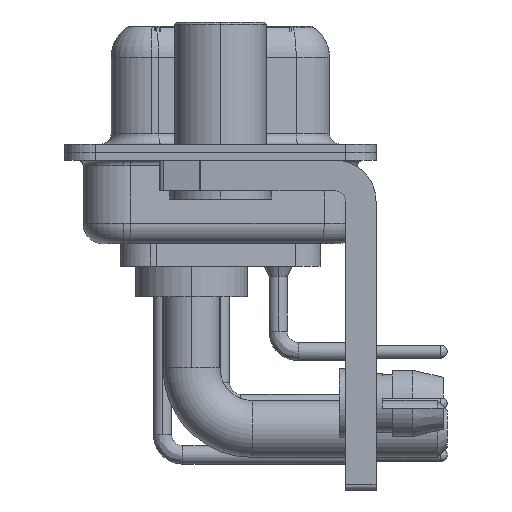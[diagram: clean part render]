
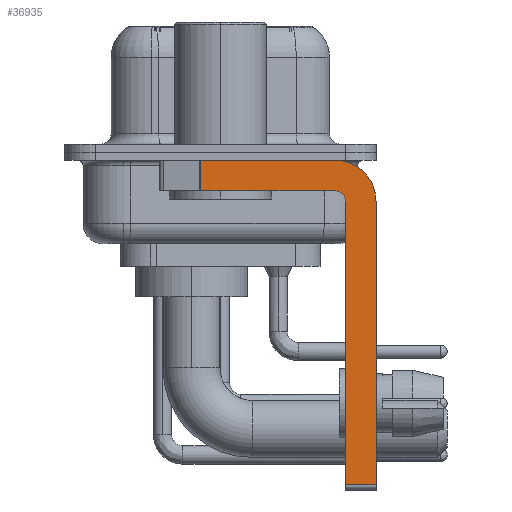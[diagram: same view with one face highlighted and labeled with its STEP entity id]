
A CAD part, left-side view. The second image highlights one B-rep face of the part: STEP entity #36935.
In plain terms, the highlighted planar face has unit normal (-1, 0, 0).
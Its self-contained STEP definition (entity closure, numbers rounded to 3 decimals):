
#1635 = VERTEX_POINT ( 'NONE', #21476 ) ;
#2178 = CARTESIAN_POINT ( 'NONE',  ( -2.9, -5.65, -2.4 ) ) ;
#2649 = DIRECTION ( 'NONE',  ( 0., 0., 1. ) ) ;
#4287 = VERTEX_POINT ( 'NONE', #17527 ) ;
#4648 = CARTESIAN_POINT ( 'NONE',  ( -2.9, -5.65, -16.35 ) ) ;
#6298 = EDGE_CURVE ( 'NONE', #4287, #22610, #14163, .T. ) ;
#6787 = EDGE_LOOP ( 'NONE', ( #34206, #25118, #25691, #21799, #35292, #10606, #28775, #34054 ) ) ;
#6945 = VECTOR ( 'NONE', #35707, 1000. ) ;
#9148 = CARTESIAN_POINT ( 'NONE',  ( -2.9, 0.978, -1.9 ) ) ;
#9877 = VECTOR ( 'NONE', #15111, 1000. ) ;
#10360 = CARTESIAN_POINT ( 'NONE',  ( -2.9, -7.65, -2.4 ) ) ;
#10606 = ORIENTED_EDGE ( 'NONE', *, *, #32240, .T. ) ;
#10685 = DIRECTION ( 'NONE',  ( -1., 0., 0. ) ) ;
#11416 = DIRECTION ( 'NONE',  ( 0., 0., -1. ) ) ;
#12202 = LINE ( 'NONE', #23993, #6945 ) ;
#12216 = CARTESIAN_POINT ( 'NONE',  ( -2.9, 0.978, -0.4 ) ) ;
#13278 = DIRECTION ( 'NONE',  ( 0., 0., -1. ) ) ;
#13971 = DIRECTION ( 'NONE',  ( 0., 0., 1. ) ) ;
#14163 = CIRCLE ( 'NONE', #35705, 2. ) ;
#14767 = LINE ( 'NONE', #26556, #30332 ) ;
#15111 = DIRECTION ( 'NONE',  ( 0., 0., -1. ) ) ;
#17416 = DIRECTION ( 'NONE',  ( 1., 0., 0. ) ) ;
#17527 = CARTESIAN_POINT ( 'NONE',  ( -2.9, -5.65, -0.4 ) ) ;
#17726 = VECTOR ( 'NONE', #28205, 1000. ) ;
#18055 = VECTOR ( 'NONE', #33056, 1000. ) ;
#18095 = LINE ( 'NONE', #29080, #20779 ) ;
#18765 = LINE ( 'NONE', #24763, #9877 ) ;
#19242 = CARTESIAN_POINT ( 'NONE',  ( -2.9, 0.978, -1.9 ) ) ;
#19274 = DIRECTION ( 'NONE',  ( 1., 0., 0. ) ) ;
#19336 = LINE ( 'NONE', #4648, #17726 ) ;
#20779 = VECTOR ( 'NONE', #2649, 1000. ) ;
#21402 = CARTESIAN_POINT ( 'NONE',  ( -2.9, -5.65, -2.4 ) ) ;
#21476 = CARTESIAN_POINT ( 'NONE',  ( -2.9, -6.15, -2.4 ) ) ;
#21799 = ORIENTED_EDGE ( 'NONE', *, *, #23094, .F. ) ;
#21969 = EDGE_CURVE ( 'NONE', #22610, #23351, #18765, .T. ) ;
#22610 = VERTEX_POINT ( 'NONE', #10360 ) ;
#23094 = EDGE_CURVE ( 'NONE', #1635, #34619, #24151, .T. ) ;
#23351 = VERTEX_POINT ( 'NONE', #30311 ) ;
#23766 = EDGE_CURVE ( 'NONE', #30049, #24838, #33240, .T. ) ;
#23993 = CARTESIAN_POINT ( 'NONE',  ( -2.9, -5.65, -1.9 ) ) ;
#24151 = CIRCLE ( 'NONE', #31540, 0.5 ) ;
#24278 = EDGE_CURVE ( 'NONE', #34619, #24838, #12202, .T. ) ;
#24763 = CARTESIAN_POINT ( 'NONE',  ( -2.9, -7.65, -2.4 ) ) ;
#24838 = VERTEX_POINT ( 'NONE', #19242 ) ;
#25118 = ORIENTED_EDGE ( 'NONE', *, *, #23766, .T. ) ;
#25128 = EDGE_CURVE ( 'NONE', #30049, #4287, #14767, .T. ) ;
#25691 = ORIENTED_EDGE ( 'NONE', *, *, #24278, .F. ) ;
#25772 = CARTESIAN_POINT ( 'NONE',  ( -2.9, -5.65, -2.4 ) ) ;
#26306 = PLANE ( 'NONE',  #35783 ) ;
#26556 = CARTESIAN_POINT ( 'NONE',  ( -2.9, 3., -0.4 ) ) ;
#28205 = DIRECTION ( 'NONE',  ( 0., -1., 0. ) ) ;
#28775 = ORIENTED_EDGE ( 'NONE', *, *, #21969, .F. ) ;
#29080 = CARTESIAN_POINT ( 'NONE',  ( -2.9, -6.15, -16.6 ) ) ;
#30049 = VERTEX_POINT ( 'NONE', #12216 ) ;
#30311 = CARTESIAN_POINT ( 'NONE',  ( -2.9, -7.65, -16.35 ) ) ;
#30332 = VECTOR ( 'NONE', #34821, 1000. ) ;
#31429 = CARTESIAN_POINT ( 'NONE',  ( -2.9, -5.65, -1.9 ) ) ;
#31540 = AXIS2_PLACEMENT_3D ( 'NONE', #25772, #10685, #13971 ) ;
#31572 = EDGE_CURVE ( 'NONE', #34248, #1635, #18095, .T. ) ;
#32240 = EDGE_CURVE ( 'NONE', #34248, #23351, #19336, .T. ) ;
#32384 = CARTESIAN_POINT ( 'NONE',  ( -2.9, -6.15, -16.35 ) ) ;
#33056 = DIRECTION ( 'NONE',  ( 0., 0., -1. ) ) ;
#33240 = LINE ( 'NONE', #9148, #18055 ) ;
#34054 = ORIENTED_EDGE ( 'NONE', *, *, #6298, .F. ) ;
#34206 = ORIENTED_EDGE ( 'NONE', *, *, #25128, .F. ) ;
#34248 = VERTEX_POINT ( 'NONE', #32384 ) ;
#34619 = VERTEX_POINT ( 'NONE', #31429 ) ;
#34746 = FACE_OUTER_BOUND ( 'NONE', #6787, .T. ) ;
#34821 = DIRECTION ( 'NONE',  ( 0., -1., 0. ) ) ;
#35292 = ORIENTED_EDGE ( 'NONE', *, *, #31572, .F. ) ;
#35705 = AXIS2_PLACEMENT_3D ( 'NONE', #21402, #19274, #13278 ) ;
#35707 = DIRECTION ( 'NONE',  ( 0., 1., 0. ) ) ;
#35783 = AXIS2_PLACEMENT_3D ( 'NONE', #2178, #17416, #11416 ) ;
#36935 = ADVANCED_FACE ( 'NONE', ( #34746 ), #26306, .F. ) ;
